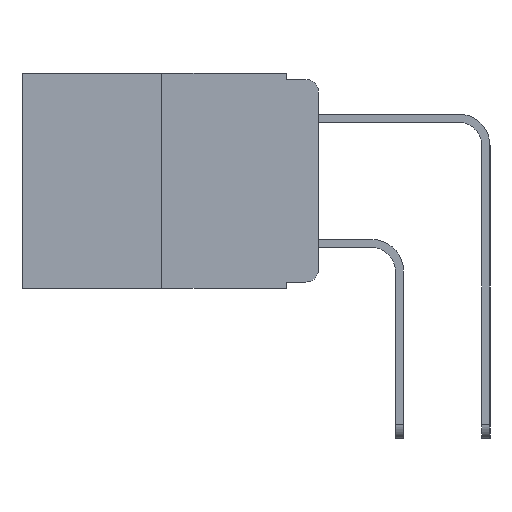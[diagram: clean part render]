
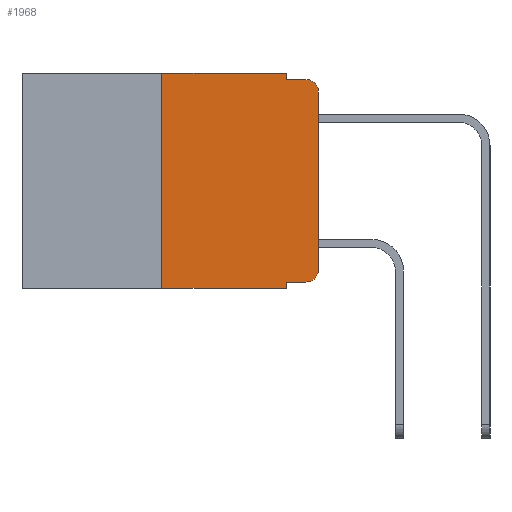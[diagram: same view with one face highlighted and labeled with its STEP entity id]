
A CAD part, left-side view. The second image highlights one B-rep face of the part: STEP entity #1968.
In plain terms, the highlighted planar face has unit normal (-1, 0, 0).
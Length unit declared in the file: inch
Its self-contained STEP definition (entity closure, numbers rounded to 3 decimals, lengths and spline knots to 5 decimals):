
#34 = ORIENTED_EDGE ( 'NONE', *, *, #3594, .T. ) ;
#207 = ORIENTED_EDGE ( 'NONE', *, *, #3563, .F. ) ;
#484 = EDGE_LOOP ( 'NONE', ( #542, #1118, #1052, #207, #796, #803, #1668, #1814, #4808, #34 ) ) ;
#542 = ORIENTED_EDGE ( 'NONE', *, *, #3537, .T. ) ;
#636 = CARTESIAN_POINT ( 'NONE',  ( 0., 0.02, -0.333 ) ) ;
#796 = ORIENTED_EDGE ( 'NONE', *, *, #1530, .F. ) ;
#803 = ORIENTED_EDGE ( 'NONE', *, *, #3566, .F. ) ;
#1052 = ORIENTED_EDGE ( 'NONE', *, *, #3544, .F. ) ;
#1118 = ORIENTED_EDGE ( 'NONE', *, *, #3538, .T. ) ;
#1171 = VERTEX_POINT ( 'NONE', #636 ) ;
#1301 = DIRECTION ( 'NONE',  ( 0., -1., 0. ) ) ;
#1369 = CARTESIAN_POINT ( 'NONE',  ( 0., 0.02, -0.03 ) ) ;
#1436 = CARTESIAN_POINT ( 'NONE',  ( 0., 0.051, 0. ) ) ;
#1530 = EDGE_CURVE ( 'NONE', #12634, #12374, #2817, .T. ) ;
#1556 = VECTOR ( 'NONE', #7979, 39.37008 ) ;
#1668 = ORIENTED_EDGE ( 'NONE', *, *, #2608, .T. ) ;
#1814 = ORIENTED_EDGE ( 'NONE', *, *, #3571, .F. ) ;
#1956 = LINE ( 'NONE', #5019, #9940 ) ;
#1968 = ADVANCED_FACE ( 'NONE', ( #10735 ), #6822, .F. ) ;
#2003 = CARTESIAN_POINT ( 'NONE',  ( 0., 0.25, 0. ) ) ;
#2371 = LINE ( 'NONE', #9882, #7706 ) ;
#2608 = EDGE_CURVE ( 'NONE', #5550, #11242, #11095, .T. ) ;
#2705 = DIRECTION ( 'NONE',  ( 0., 0., -1. ) ) ;
#2786 = LINE ( 'NONE', #5961, #8287 ) ;
#2817 = LINE ( 'NONE', #8800, #6049 ) ;
#2872 = CARTESIAN_POINT ( 'NONE',  ( 0., 0.02, -0.313 ) ) ;
#3537 = EDGE_CURVE ( 'NONE', #5673, #6152, #2786, .T. ) ;
#3538 = EDGE_CURVE ( 'NONE', #6152, #6026, #10740, .T. ) ;
#3544 = EDGE_CURVE ( 'NONE', #4068, #6026, #13008, .T. ) ;
#3563 = EDGE_CURVE ( 'NONE', #12374, #4068, #2371, .T. ) ;
#3566 = EDGE_CURVE ( 'NONE', #5550, #12634, #1956, .T. ) ;
#3571 = EDGE_CURVE ( 'NONE', #5929, #11242, #10208, .T. ) ;
#3592 = EDGE_CURVE ( 'NONE', #5929, #1171, #9654, .T. ) ;
#3594 = EDGE_CURVE ( 'NONE', #1171, #5673, #12224, .T. ) ;
#3810 = AXIS2_PLACEMENT_3D ( 'NONE', #1369, #8892, #2705 ) ;
#3914 = DIRECTION ( 'NONE',  ( 0., -1., 0. ) ) ;
#4054 = DIRECTION ( 'NONE',  ( 0., 0., -1. ) ) ;
#4068 = VERTEX_POINT ( 'NONE', #6625 ) ;
#4411 = VECTOR ( 'NONE', #5071, 39.37008 ) ;
#4808 = ORIENTED_EDGE ( 'NONE', *, *, #3592, .T. ) ;
#5019 = CARTESIAN_POINT ( 'NONE',  ( 0., 0.25, 0. ) ) ;
#5071 = DIRECTION ( 'NONE',  ( 0., -1., 0. ) ) ;
#5300 = CARTESIAN_POINT ( 'NONE',  ( 0., 0., -0.313 ) ) ;
#5388 = VECTOR ( 'NONE', #3914, 39.37008 ) ;
#5550 = VERTEX_POINT ( 'NONE', #11655 ) ;
#5673 = VERTEX_POINT ( 'NONE', #5300 ) ;
#5929 = VERTEX_POINT ( 'NONE', #8509 ) ;
#5961 = CARTESIAN_POINT ( 'NONE',  ( 0., 0., 0. ) ) ;
#6002 = DIRECTION ( 'NONE',  ( 0., 0., -1. ) ) ;
#6026 = VERTEX_POINT ( 'NONE', #12177 ) ;
#6047 = DIRECTION ( 'NONE',  ( 0., 0., 1. ) ) ;
#6049 = VECTOR ( 'NONE', #8342, 39.37008 ) ;
#6152 = VERTEX_POINT ( 'NONE', #7741 ) ;
#6497 = CARTESIAN_POINT ( 'NONE',  ( 0., 0.051, -0.343 ) ) ;
#6579 = AXIS2_PLACEMENT_3D ( 'NONE', #2872, #9959, #4054 ) ;
#6625 = CARTESIAN_POINT ( 'NONE',  ( 0., 0.051, -0.01 ) ) ;
#6672 = DIRECTION ( 'NONE',  ( 0., 0., -1. ) ) ;
#6702 = DIRECTION ( 'NONE',  ( 1., 0., 0. ) ) ;
#6783 = CARTESIAN_POINT ( 'NONE',  ( 0., 0.473, 0. ) ) ;
#6822 = PLANE ( 'NONE',  #9371 ) ;
#7706 = VECTOR ( 'NONE', #6002, 39.37008 ) ;
#7741 = CARTESIAN_POINT ( 'NONE',  ( 0., 0., -0.03 ) ) ;
#7979 = DIRECTION ( 'NONE',  ( 0., 0., -1. ) ) ;
#8287 = VECTOR ( 'NONE', #12395, 39.37008 ) ;
#8342 = DIRECTION ( 'NONE',  ( 0., -1., 0. ) ) ;
#8509 = CARTESIAN_POINT ( 'NONE',  ( 0., 0.051, -0.333 ) ) ;
#8800 = CARTESIAN_POINT ( 'NONE',  ( 0., 0.473, 0. ) ) ;
#8808 = CARTESIAN_POINT ( 'NONE',  ( 0., 0.473, -0.343 ) ) ;
#8892 = DIRECTION ( 'NONE',  ( -1., 0., 0. ) ) ;
#9371 = AXIS2_PLACEMENT_3D ( 'NONE', #6783, #6702, #6672 ) ;
#9654 = LINE ( 'NONE', #10779, #4411 ) ;
#9835 = CARTESIAN_POINT ( 'NONE',  ( 0., 0.051, -0.01 ) ) ;
#9882 = CARTESIAN_POINT ( 'NONE',  ( 0., 0.051, 0. ) ) ;
#9940 = VECTOR ( 'NONE', #6047, 39.37008 ) ;
#9959 = DIRECTION ( 'NONE',  ( -1., 0., 0. ) ) ;
#10208 = LINE ( 'NONE', #1436, #1556 ) ;
#10735 = FACE_OUTER_BOUND ( 'NONE', #484, .T. ) ;
#10740 = CIRCLE ( 'NONE', #3810, 0.02 ) ;
#10779 = CARTESIAN_POINT ( 'NONE',  ( 0., 0.051, -0.333 ) ) ;
#10836 = VECTOR ( 'NONE', #1301, 39.37008 ) ;
#11095 = LINE ( 'NONE', #8808, #10836 ) ;
#11242 = VERTEX_POINT ( 'NONE', #6497 ) ;
#11571 = CARTESIAN_POINT ( 'NONE',  ( 0., 0.051, 0. ) ) ;
#11655 = CARTESIAN_POINT ( 'NONE',  ( 0., 0.25, -0.343 ) ) ;
#12177 = CARTESIAN_POINT ( 'NONE',  ( 0., 0.02, -0.01 ) ) ;
#12224 = CIRCLE ( 'NONE', #6579, 0.02 ) ;
#12374 = VERTEX_POINT ( 'NONE', #11571 ) ;
#12395 = DIRECTION ( 'NONE',  ( 0., 0., 1. ) ) ;
#12634 = VERTEX_POINT ( 'NONE', #2003 ) ;
#13008 = LINE ( 'NONE', #9835, #5388 ) ;
